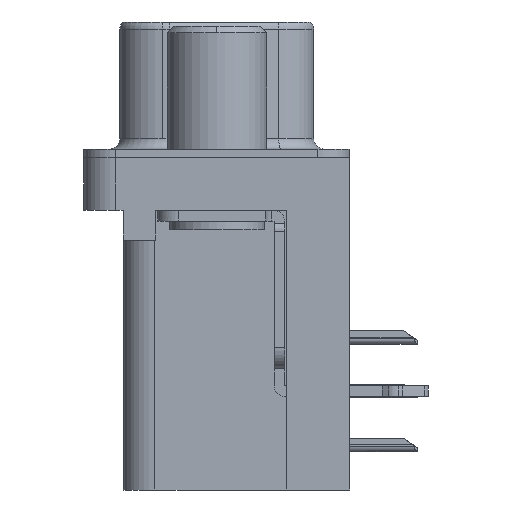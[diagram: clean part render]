
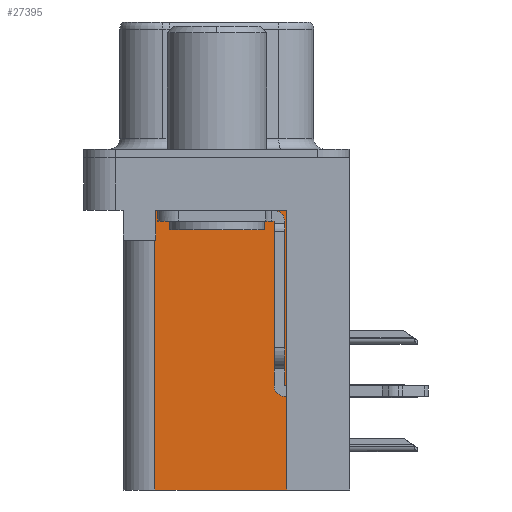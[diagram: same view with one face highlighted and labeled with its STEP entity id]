
A CAD part, left-side view. The second image highlights one B-rep face of the part: STEP entity #27395.
In plain terms, the highlighted planar face has unit normal (-1, 0, 0).
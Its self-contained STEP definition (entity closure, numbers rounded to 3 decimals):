
#2223 = DIRECTION ( 'NONE',  ( 0., 1., 0. ) ) ;
#3139 = VECTOR ( 'NONE', #26406, 1000. ) ;
#3668 = DIRECTION ( 'NONE',  ( 0., 0., 1. ) ) ;
#4165 = EDGE_CURVE ( 'NONE', #29865, #9282, #11793, .T. ) ;
#4282 = CARTESIAN_POINT ( 'NONE',  ( 3.79, -3.295, -2.5 ) ) ;
#4434 = EDGE_CURVE ( 'NONE', #9282, #35735, #26968, .T. ) ;
#4582 = ORIENTED_EDGE ( 'NONE', *, *, #4827, .T. ) ;
#4827 = EDGE_CURVE ( 'NONE', #35735, #9115, #35029, .T. ) ;
#7629 = CARTESIAN_POINT ( 'NONE',  ( 3.79, -3.295, -15.7 ) ) ;
#8219 = LINE ( 'NONE', #23050, #21903 ) ;
#8541 = CARTESIAN_POINT ( 'NONE',  ( 3.79, 2.895, -3.9 ) ) ;
#9115 = VERTEX_POINT ( 'NONE', #20563 ) ;
#9282 = VERTEX_POINT ( 'NONE', #35022 ) ;
#9284 = PLANE ( 'NONE',  #25424 ) ;
#9548 = EDGE_CURVE ( 'NONE', #18997, #9115, #8219, .T. ) ;
#9842 = EDGE_CURVE ( 'NONE', #32002, #18997, #19784, .T. ) ;
#9892 = EDGE_CURVE ( 'NONE', #32002, #29865, #34285, .T. ) ;
#10041 = VECTOR ( 'NONE', #16672, 1000. ) ;
#10509 = ORIENTED_EDGE ( 'NONE', *, *, #9548, .F. ) ;
#11231 = CARTESIAN_POINT ( 'NONE',  ( 3.79, 0., -3.9 ) ) ;
#11793 = LINE ( 'NONE', #4282, #3139 ) ;
#12085 = CARTESIAN_POINT ( 'NONE',  ( 3.79, -3.295, -15.7 ) ) ;
#12198 = DIRECTION ( 'NONE',  ( 1., 0., 0. ) ) ;
#12356 = ORIENTED_EDGE ( 'NONE', *, *, #9892, .T. ) ;
#13891 = CARTESIAN_POINT ( 'NONE',  ( 3.79, -3.295, -2.5 ) ) ;
#14198 = DIRECTION ( 'NONE',  ( 0., 0., -1. ) ) ;
#16672 = DIRECTION ( 'NONE',  ( 0., 0., 1. ) ) ;
#18997 = VERTEX_POINT ( 'NONE', #20279 ) ;
#19690 = VECTOR ( 'NONE', #14198, 1000. ) ;
#19784 = LINE ( 'NONE', #35341, #26200 ) ;
#20279 = CARTESIAN_POINT ( 'NONE',  ( 3.79, 2.925, -15.7 ) ) ;
#20563 = CARTESIAN_POINT ( 'NONE',  ( 3.79, 2.925, -3.9 ) ) ;
#21903 = VECTOR ( 'NONE', #3668, 1000. ) ;
#23050 = CARTESIAN_POINT ( 'NONE',  ( 3.79, 2.925, -15.7 ) ) ;
#25424 = AXIS2_PLACEMENT_3D ( 'NONE', #12085, #12198, #31091 ) ;
#26200 = VECTOR ( 'NONE', #2223, 1000. ) ;
#26406 = DIRECTION ( 'NONE',  ( 0., 1., 0. ) ) ;
#26736 = FACE_OUTER_BOUND ( 'NONE', #35168, .T. ) ;
#26968 = LINE ( 'NONE', #8541, #19690 ) ;
#27395 = ADVANCED_FACE ( 'NONE', ( #26736 ), #9284, .F. ) ;
#27420 = DIRECTION ( 'NONE',  ( 0., 1., 0. ) ) ;
#27766 = VECTOR ( 'NONE', #27420, 1000. ) ;
#28454 = ORIENTED_EDGE ( 'NONE', *, *, #4165, .T. ) ;
#29865 = VERTEX_POINT ( 'NONE', #13891 ) ;
#30395 = CARTESIAN_POINT ( 'NONE',  ( 3.79, 2.895, -3.9 ) ) ;
#30454 = ORIENTED_EDGE ( 'NONE', *, *, #4434, .T. ) ;
#31091 = DIRECTION ( 'NONE',  ( 0., 0., -1. ) ) ;
#32002 = VERTEX_POINT ( 'NONE', #7629 ) ;
#32953 = CARTESIAN_POINT ( 'NONE',  ( 3.79, -3.295, -15.7 ) ) ;
#33401 = ORIENTED_EDGE ( 'NONE', *, *, #9842, .F. ) ;
#34285 = LINE ( 'NONE', #32953, #10041 ) ;
#35022 = CARTESIAN_POINT ( 'NONE',  ( 3.79, 2.895, -2.5 ) ) ;
#35029 = LINE ( 'NONE', #11231, #27766 ) ;
#35168 = EDGE_LOOP ( 'NONE', ( #28454, #30454, #4582, #10509, #33401, #12356 ) ) ;
#35341 = CARTESIAN_POINT ( 'NONE',  ( 3.79, -3.295, -15.7 ) ) ;
#35735 = VERTEX_POINT ( 'NONE', #30395 ) ;
